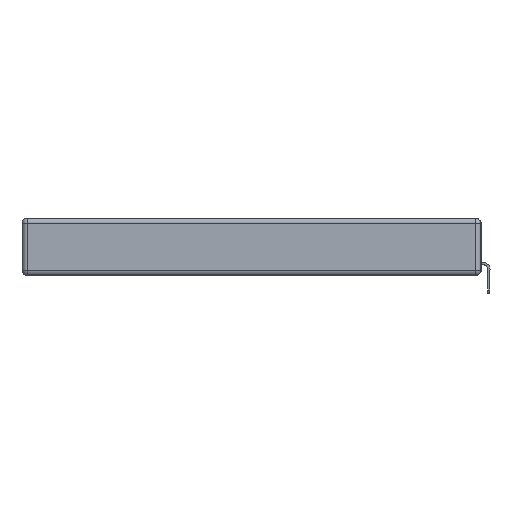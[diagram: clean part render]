
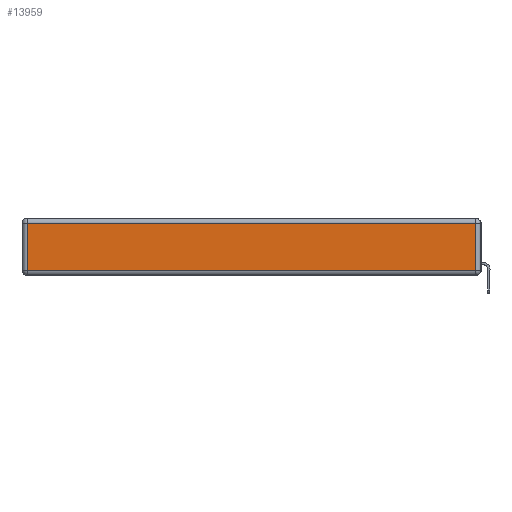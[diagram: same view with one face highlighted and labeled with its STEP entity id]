
A CAD part, left-side view. The second image highlights one B-rep face of the part: STEP entity #13959.
In plain terms, the highlighted planar face has unit normal (-1, 0, 0).
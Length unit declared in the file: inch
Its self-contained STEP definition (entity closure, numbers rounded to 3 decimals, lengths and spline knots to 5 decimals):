
#1252 = LINE ( 'NONE', #5682, #9791 ) ;
#2070 = CARTESIAN_POINT ( 'NONE',  ( 0., 2.72, -0.313 ) ) ;
#2552 = CARTESIAN_POINT ( 'NONE',  ( 0., 2.72, -0.343 ) ) ;
#3302 = VECTOR ( 'NONE', #14095, 39.37008 ) ;
#4415 = ORIENTED_EDGE ( 'NONE', *, *, #4954, .T. ) ;
#4490 = EDGE_CURVE ( 'NONE', #13808, #8755, #13337, .T. ) ;
#4954 = EDGE_CURVE ( 'NONE', #7565, #15898, #8642, .T. ) ;
#5682 = CARTESIAN_POINT ( 'NONE',  ( 0., 2.75, -0.03 ) ) ;
#6432 = VECTOR ( 'NONE', #16216, 39.37008 ) ;
#6582 = ORIENTED_EDGE ( 'NONE', *, *, #4490, .T. ) ;
#6685 = EDGE_CURVE ( 'NONE', #15898, #13808, #1252, .T. ) ;
#6889 = DIRECTION ( 'NONE',  ( 0., 1., 0. ) ) ;
#7269 = PLANE ( 'NONE',  #12817 ) ;
#7565 = VERTEX_POINT ( 'NONE', #12509 ) ;
#8290 = ORIENTED_EDGE ( 'NONE', *, *, #6685, .T. ) ;
#8642 = LINE ( 'NONE', #12482, #15331 ) ;
#8755 = VERTEX_POINT ( 'NONE', #2070 ) ;
#9791 = VECTOR ( 'NONE', #6889, 39.37008 ) ;
#9828 = CARTESIAN_POINT ( 'NONE',  ( 0., 0., -0.343 ) ) ;
#9891 = DIRECTION ( 'NONE',  ( 0., 0., 1. ) ) ;
#9897 = EDGE_LOOP ( 'NONE', ( #14723, #4415, #8290, #6582 ) ) ;
#10424 = FACE_OUTER_BOUND ( 'NONE', #9897, .T. ) ;
#10738 = CARTESIAN_POINT ( 'NONE',  ( 0., 2.72, -0.03 ) ) ;
#12341 = DIRECTION ( 'NONE',  ( -1., 0., 0. ) ) ;
#12482 = CARTESIAN_POINT ( 'NONE',  ( 0., 0.03, -0.343 ) ) ;
#12509 = CARTESIAN_POINT ( 'NONE',  ( 0., 0.03, -0.313 ) ) ;
#12817 = AXIS2_PLACEMENT_3D ( 'NONE', #9828, #12341, #9891 ) ;
#13337 = LINE ( 'NONE', #2552, #6432 ) ;
#13808 = VERTEX_POINT ( 'NONE', #10738 ) ;
#13959 = ADVANCED_FACE ( 'NONE', ( #10424 ), #7269, .T. ) ;
#14080 = LINE ( 'NONE', #14160, #3302 ) ;
#14095 = DIRECTION ( 'NONE',  ( 0., -1., 0. ) ) ;
#14160 = CARTESIAN_POINT ( 'NONE',  ( 0., 0., -0.313 ) ) ;
#14603 = EDGE_CURVE ( 'NONE', #8755, #7565, #14080, .T. ) ;
#14723 = ORIENTED_EDGE ( 'NONE', *, *, #14603, .T. ) ;
#15331 = VECTOR ( 'NONE', #16351, 39.37008 ) ;
#15898 = VERTEX_POINT ( 'NONE', #16409 ) ;
#16216 = DIRECTION ( 'NONE',  ( 0., 0., -1. ) ) ;
#16351 = DIRECTION ( 'NONE',  ( 0., 0., 1. ) ) ;
#16409 = CARTESIAN_POINT ( 'NONE',  ( 0., 0.03, -0.03 ) ) ;
